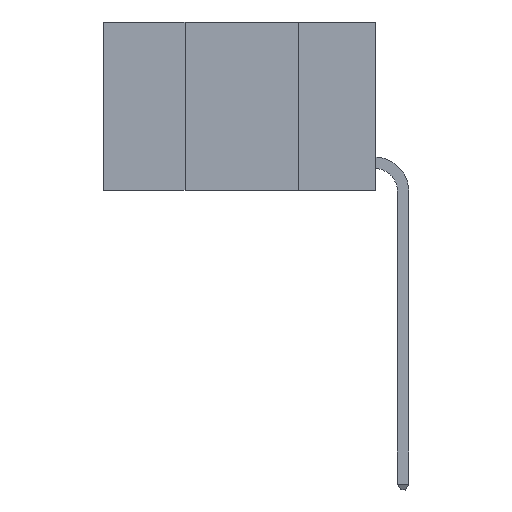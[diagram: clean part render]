
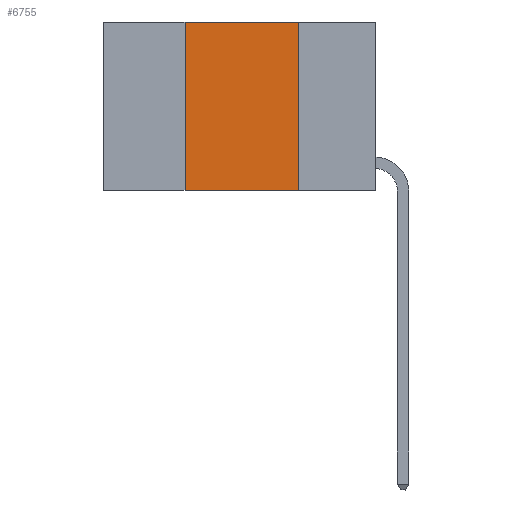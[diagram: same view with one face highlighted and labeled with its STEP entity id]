
A CAD part, left-side view. The second image highlights one B-rep face of the part: STEP entity #6755.
In plain terms, the highlighted planar face has unit normal (-1, 0, 0).
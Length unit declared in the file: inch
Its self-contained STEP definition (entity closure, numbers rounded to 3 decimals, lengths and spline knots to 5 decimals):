
#59 = CARTESIAN_POINT ( 'NONE',  ( 0., 0.42, 0. ) ) ;
#813 = VECTOR ( 'NONE', #4372, 39.37008 ) ;
#1311 = LINE ( 'NONE', #19708, #813 ) ;
#2011 = VECTOR ( 'NONE', #17881, 39.37008 ) ;
#2055 = EDGE_CURVE ( 'NONE', #3979, #16204, #1311, .T. ) ;
#2469 = CARTESIAN_POINT ( 'NONE',  ( 0., 0.17, -0.37 ) ) ;
#2526 = DIRECTION ( 'NONE',  ( 1., 0., 0. ) ) ;
#2719 = EDGE_CURVE ( 'NONE', #3979, #14552, #18439, .T. ) ;
#3819 = VECTOR ( 'NONE', #4229, 39.37008 ) ;
#3979 = VERTEX_POINT ( 'NONE', #4571 ) ;
#4229 = DIRECTION ( 'NONE',  ( 0., -1., 0. ) ) ;
#4299 = LINE ( 'NONE', #19631, #3819 ) ;
#4372 = DIRECTION ( 'NONE',  ( 0., -1., 0. ) ) ;
#4399 = EDGE_CURVE ( 'NONE', #17849, #16204, #19848, .T. ) ;
#4571 = CARTESIAN_POINT ( 'NONE',  ( 0., 0.42, -0.37 ) ) ;
#4657 = ORIENTED_EDGE ( 'NONE', *, *, #10926, .F. ) ;
#6291 = ORIENTED_EDGE ( 'NONE', *, *, #2055, .T. ) ;
#6755 = ADVANCED_FACE ( 'NONE', ( #9416 ), #8669, .F. ) ;
#7109 = CARTESIAN_POINT ( 'NONE',  ( 0., 0.17, 0. ) ) ;
#7337 = CARTESIAN_POINT ( 'NONE',  ( 0., 0.17, 0. ) ) ;
#7684 = EDGE_LOOP ( 'NONE', ( #9439, #4657, #10843, #6291 ) ) ;
#8669 = PLANE ( 'NONE',  #10373 ) ;
#9416 = FACE_OUTER_BOUND ( 'NONE', #7684, .T. ) ;
#9439 = ORIENTED_EDGE ( 'NONE', *, *, #4399, .F. ) ;
#10373 = AXIS2_PLACEMENT_3D ( 'NONE', #11771, #2526, #13301 ) ;
#10843 = ORIENTED_EDGE ( 'NONE', *, *, #2719, .F. ) ;
#10926 = EDGE_CURVE ( 'NONE', #14552, #17849, #4299, .T. ) ;
#11771 = CARTESIAN_POINT ( 'NONE',  ( 0., 0.6, 0. ) ) ;
#12052 = CARTESIAN_POINT ( 'NONE',  ( 0., 0.42, 0. ) ) ;
#13301 = DIRECTION ( 'NONE',  ( 0., 0., -1. ) ) ;
#14365 = VECTOR ( 'NONE', #15545, 39.37008 ) ;
#14552 = VERTEX_POINT ( 'NONE', #12052 ) ;
#15545 = DIRECTION ( 'NONE',  ( 0., 0., 1. ) ) ;
#16204 = VERTEX_POINT ( 'NONE', #2469 ) ;
#17849 = VERTEX_POINT ( 'NONE', #7337 ) ;
#17881 = DIRECTION ( 'NONE',  ( 0., 0., -1. ) ) ;
#18439 = LINE ( 'NONE', #59, #14365 ) ;
#19631 = CARTESIAN_POINT ( 'NONE',  ( 0., 0.6, 0. ) ) ;
#19708 = CARTESIAN_POINT ( 'NONE',  ( 0., 0.6, -0.37 ) ) ;
#19848 = LINE ( 'NONE', #7109, #2011 ) ;
